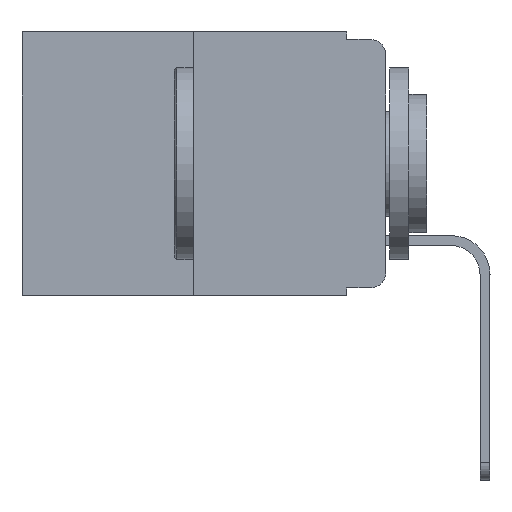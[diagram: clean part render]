
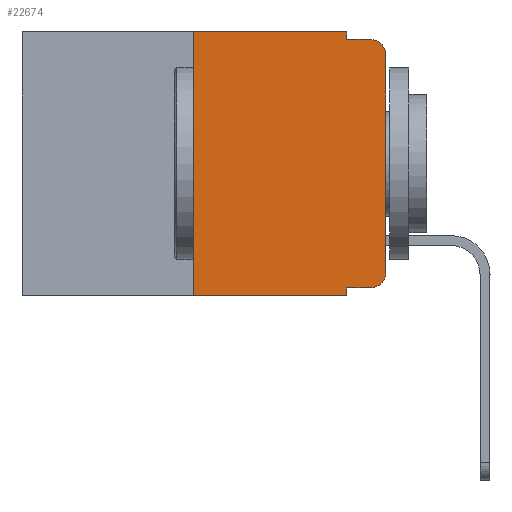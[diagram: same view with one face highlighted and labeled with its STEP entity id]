
A CAD part, left-side view. The second image highlights one B-rep face of the part: STEP entity #22674.
In plain terms, the highlighted planar face has unit normal (-1, 0, 0).
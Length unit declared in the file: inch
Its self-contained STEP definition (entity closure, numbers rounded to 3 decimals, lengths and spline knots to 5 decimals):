
#401 = CARTESIAN_POINT ( 'NONE',  ( 0., 0.051, 0. ) ) ;
#455 = VERTEX_POINT ( 'NONE', #17918 ) ;
#509 = EDGE_CURVE ( 'NONE', #17882, #11480, #8790, .T. ) ;
#748 = CARTESIAN_POINT ( 'NONE',  ( 0., 0.473, -0.343 ) ) ;
#1475 = CARTESIAN_POINT ( 'NONE',  ( 0., 0.051, -0.343 ) ) ;
#1497 = DIRECTION ( 'NONE',  ( 0., 0., -1. ) ) ;
#1505 = CARTESIAN_POINT ( 'NONE',  ( 0., 0.25, -0.343 ) ) ;
#1814 = CARTESIAN_POINT ( 'NONE',  ( 0., 0.051, 0. ) ) ;
#2085 = DIRECTION ( 'NONE',  ( 0., -1., 0. ) ) ;
#2862 = VERTEX_POINT ( 'NONE', #5260 ) ;
#2915 = LINE ( 'NONE', #9402, #25045 ) ;
#3728 = LINE ( 'NONE', #23981, #22711 ) ;
#3894 = CARTESIAN_POINT ( 'NONE',  ( 0., 0., -0.03 ) ) ;
#3904 = LINE ( 'NONE', #22445, #26014 ) ;
#3957 = VECTOR ( 'NONE', #2085, 39.37008 ) ;
#4106 = CARTESIAN_POINT ( 'NONE',  ( 0., 0.473, 0. ) ) ;
#4764 = DIRECTION ( 'NONE',  ( 0., 0., -1. ) ) ;
#5246 = EDGE_CURVE ( 'NONE', #13898, #22448, #5423, .T. ) ;
#5260 = CARTESIAN_POINT ( 'NONE',  ( 0., 0., -0.313 ) ) ;
#5423 = CIRCLE ( 'NONE', #10042, 0.02 ) ;
#6506 = DIRECTION ( 'NONE',  ( 0., 0., -1. ) ) ;
#6697 = ORIENTED_EDGE ( 'NONE', *, *, #5246, .T. ) ;
#7499 = CARTESIAN_POINT ( 'NONE',  ( 0., 0.051, -0.01 ) ) ;
#7820 = CIRCLE ( 'NONE', #23496, 0.02 ) ;
#8172 = ORIENTED_EDGE ( 'NONE', *, *, #22832, .F. ) ;
#8251 = CARTESIAN_POINT ( 'NONE',  ( 0., 0.051, 0. ) ) ;
#8256 = CARTESIAN_POINT ( 'NONE',  ( 0., 0.473, 0. ) ) ;
#8559 = VECTOR ( 'NONE', #11066, 39.37008 ) ;
#8566 = ORIENTED_EDGE ( 'NONE', *, *, #509, .F. ) ;
#8790 = LINE ( 'NONE', #1814, #14755 ) ;
#9394 = DIRECTION ( 'NONE',  ( -1., 0., 0. ) ) ;
#9402 = CARTESIAN_POINT ( 'NONE',  ( 0., 0.051, -0.333 ) ) ;
#9529 = EDGE_LOOP ( 'NONE', ( #12781, #6697, #9679, #8566, #22765, #21619, #16434, #8172, #15848, #20595 ) ) ;
#9679 = ORIENTED_EDGE ( 'NONE', *, *, #17108, .F. ) ;
#9938 = LINE ( 'NONE', #8256, #3957 ) ;
#10042 = AXIS2_PLACEMENT_3D ( 'NONE', #16833, #14787, #4764 ) ;
#11066 = DIRECTION ( 'NONE',  ( 0., -1., 0. ) ) ;
#11480 = VERTEX_POINT ( 'NONE', #7499 ) ;
#11550 = VERTEX_POINT ( 'NONE', #1505 ) ;
#11591 = CARTESIAN_POINT ( 'NONE',  ( 0., 0.02, -0.01 ) ) ;
#12319 = VERTEX_POINT ( 'NONE', #16259 ) ;
#12539 = DIRECTION ( 'NONE',  ( 0., -1., 0. ) ) ;
#12781 = ORIENTED_EDGE ( 'NONE', *, *, #15790, .T. ) ;
#13536 = DIRECTION ( 'NONE',  ( 0., -1., 0. ) ) ;
#13898 = VERTEX_POINT ( 'NONE', #3894 ) ;
#14285 = VERTEX_POINT ( 'NONE', #19459 ) ;
#14312 = LINE ( 'NONE', #748, #25738 ) ;
#14755 = VECTOR ( 'NONE', #18008, 39.37008 ) ;
#14787 = DIRECTION ( 'NONE',  ( -1., 0., 0. ) ) ;
#15075 = EDGE_CURVE ( 'NONE', #12319, #17882, #9938, .T. ) ;
#15189 = EDGE_CURVE ( 'NONE', #11550, #22516, #14312, .T. ) ;
#15790 = EDGE_CURVE ( 'NONE', #2862, #13898, #3904, .T. ) ;
#15794 = LINE ( 'NONE', #21148, #8559 ) ;
#15810 = DIRECTION ( 'NONE',  ( 0., 0., 1. ) ) ;
#15848 = ORIENTED_EDGE ( 'NONE', *, *, #16245, .T. ) ;
#16245 = EDGE_CURVE ( 'NONE', #455, #14285, #2915, .T. ) ;
#16259 = CARTESIAN_POINT ( 'NONE',  ( 0., 0.25, 0. ) ) ;
#16434 = ORIENTED_EDGE ( 'NONE', *, *, #15189, .T. ) ;
#16833 = CARTESIAN_POINT ( 'NONE',  ( 0., 0.02, -0.03 ) ) ;
#17108 = EDGE_CURVE ( 'NONE', #11480, #22448, #15794, .T. ) ;
#17882 = VERTEX_POINT ( 'NONE', #8251 ) ;
#17918 = CARTESIAN_POINT ( 'NONE',  ( 0., 0.051, -0.333 ) ) ;
#18008 = DIRECTION ( 'NONE',  ( 0., 0., -1. ) ) ;
#18885 = FACE_OUTER_BOUND ( 'NONE', #9529, .T. ) ;
#18928 = EDGE_CURVE ( 'NONE', #14285, #2862, #7820, .T. ) ;
#19457 = CARTESIAN_POINT ( 'NONE',  ( 0., 0.02, -0.313 ) ) ;
#19459 = CARTESIAN_POINT ( 'NONE',  ( 0., 0.02, -0.333 ) ) ;
#20241 = DIRECTION ( 'NONE',  ( 1., 0., 0. ) ) ;
#20405 = DIRECTION ( 'NONE',  ( 0., 0., 1. ) ) ;
#20595 = ORIENTED_EDGE ( 'NONE', *, *, #18928, .T. ) ;
#20920 = LINE ( 'NONE', #401, #25438 ) ;
#21148 = CARTESIAN_POINT ( 'NONE',  ( 0., 0.051, -0.01 ) ) ;
#21619 = ORIENTED_EDGE ( 'NONE', *, *, #22513, .F. ) ;
#22222 = PLANE ( 'NONE',  #24442 ) ;
#22445 = CARTESIAN_POINT ( 'NONE',  ( 0., 0., 0. ) ) ;
#22448 = VERTEX_POINT ( 'NONE', #11591 ) ;
#22513 = EDGE_CURVE ( 'NONE', #11550, #12319, #3728, .T. ) ;
#22516 = VERTEX_POINT ( 'NONE', #1475 ) ;
#22674 = ADVANCED_FACE ( 'NONE', ( #18885 ), #22222, .F. ) ;
#22711 = VECTOR ( 'NONE', #15810, 39.37008 ) ;
#22765 = ORIENTED_EDGE ( 'NONE', *, *, #15075, .F. ) ;
#22832 = EDGE_CURVE ( 'NONE', #455, #22516, #20920, .T. ) ;
#23496 = AXIS2_PLACEMENT_3D ( 'NONE', #19457, #9394, #1497 ) ;
#23981 = CARTESIAN_POINT ( 'NONE',  ( 0., 0.25, 0. ) ) ;
#24442 = AXIS2_PLACEMENT_3D ( 'NONE', #4106, #20241, #26001 ) ;
#25045 = VECTOR ( 'NONE', #13536, 39.37008 ) ;
#25438 = VECTOR ( 'NONE', #6506, 39.37008 ) ;
#25738 = VECTOR ( 'NONE', #12539, 39.37008 ) ;
#26001 = DIRECTION ( 'NONE',  ( 0., 0., -1. ) ) ;
#26014 = VECTOR ( 'NONE', #20405, 39.37008 ) ;
